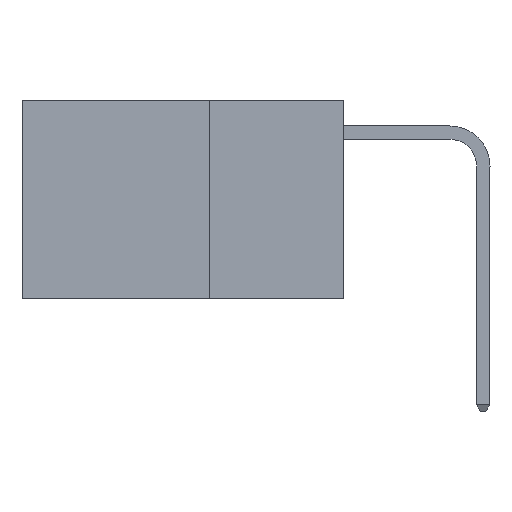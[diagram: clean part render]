
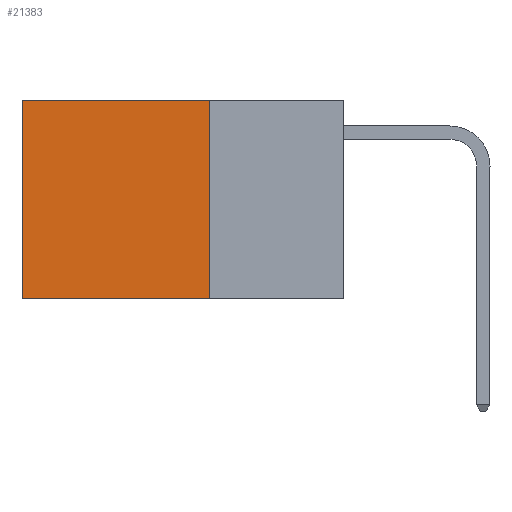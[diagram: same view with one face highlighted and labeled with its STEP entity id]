
A CAD part, left-side view. The second image highlights one B-rep face of the part: STEP entity #21383.
In plain terms, the highlighted planar face has unit normal (-1, 0, 0).
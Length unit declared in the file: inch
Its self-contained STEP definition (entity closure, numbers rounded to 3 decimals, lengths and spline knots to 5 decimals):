
#675 = LINE ( 'NONE', #19094, #1247 ) ;
#866 = FACE_OUTER_BOUND ( 'NONE', #10062, .T. ) ;
#1247 = VECTOR ( 'NONE', #19011, 39.37008 ) ;
#2782 = EDGE_CURVE ( 'NONE', #9433, #15342, #675, .T. ) ;
#2946 = ORIENTED_EDGE ( 'NONE', *, *, #17843, .T. ) ;
#3341 = ORIENTED_EDGE ( 'NONE', *, *, #5677, .T. ) ;
#3395 = CARTESIAN_POINT ( 'NONE',  ( 0.2625, 0.25, 0. ) ) ;
#3557 = LINE ( 'NONE', #5747, #4146 ) ;
#4146 = VECTOR ( 'NONE', #13062, 39.37008 ) ;
#4286 = CARTESIAN_POINT ( 'NONE',  ( 0.2625, 0.25, 0. ) ) ;
#5330 = LINE ( 'NONE', #8539, #19063 ) ;
#5677 = EDGE_CURVE ( 'NONE', #22641, #6924, #10484, .T. ) ;
#5688 = VECTOR ( 'NONE', #8988, 39.37008 ) ;
#5747 = CARTESIAN_POINT ( 'NONE',  ( 0.2625, 0.25, -0.37 ) ) ;
#5815 = AXIS2_PLACEMENT_3D ( 'NONE', #4286, #16860, #6105 ) ;
#6105 = DIRECTION ( 'NONE',  ( 0., 0., -1. ) ) ;
#6891 = CARTESIAN_POINT ( 'NONE',  ( 0.2625, 0.6, -0.37 ) ) ;
#6924 = VERTEX_POINT ( 'NONE', #6891 ) ;
#8539 = CARTESIAN_POINT ( 'NONE',  ( 0.2625, 0.25, 0. ) ) ;
#8988 = DIRECTION ( 'NONE',  ( 0., 0., -1. ) ) ;
#9433 = VERTEX_POINT ( 'NONE', #3395 ) ;
#9808 = CARTESIAN_POINT ( 'NONE',  ( 0.2625, 0.6, 0. ) ) ;
#10062 = EDGE_LOOP ( 'NONE', ( #3341, #20544, #13395, #2946 ) ) ;
#10352 = DIRECTION ( 'NONE',  ( 0., 1., 0. ) ) ;
#10484 = LINE ( 'NONE', #16151, #5688 ) ;
#12265 = CARTESIAN_POINT ( 'NONE',  ( 0.2625, 0.25, -0.37 ) ) ;
#13062 = DIRECTION ( 'NONE',  ( 0., 1., 0. ) ) ;
#13395 = ORIENTED_EDGE ( 'NONE', *, *, #2782, .F. ) ;
#15088 = PLANE ( 'NONE',  #5815 ) ;
#15342 = VERTEX_POINT ( 'NONE', #12265 ) ;
#16151 = CARTESIAN_POINT ( 'NONE',  ( 0.2625, 0.6, 0. ) ) ;
#16860 = DIRECTION ( 'NONE',  ( 1., 0., 0. ) ) ;
#17843 = EDGE_CURVE ( 'NONE', #9433, #22641, #5330, .T. ) ;
#18817 = EDGE_CURVE ( 'NONE', #15342, #6924, #3557, .T. ) ;
#19011 = DIRECTION ( 'NONE',  ( 0., 0., -1. ) ) ;
#19063 = VECTOR ( 'NONE', #10352, 39.37008 ) ;
#19094 = CARTESIAN_POINT ( 'NONE',  ( 0.2625, 0.25, 0. ) ) ;
#20544 = ORIENTED_EDGE ( 'NONE', *, *, #18817, .F. ) ;
#21383 = ADVANCED_FACE ( 'NONE', ( #866 ), #15088, .F. ) ;
#22641 = VERTEX_POINT ( 'NONE', #9808 ) ;
